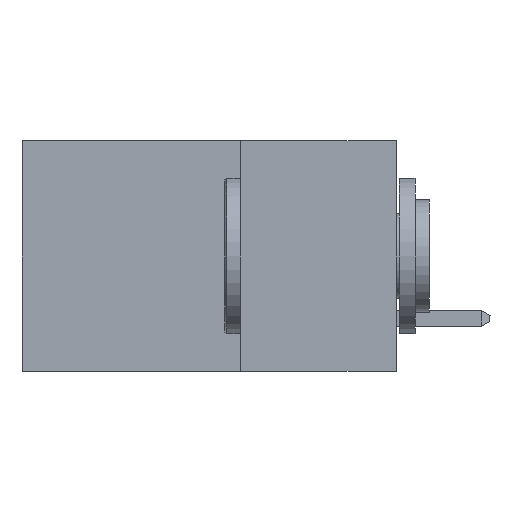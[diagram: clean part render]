
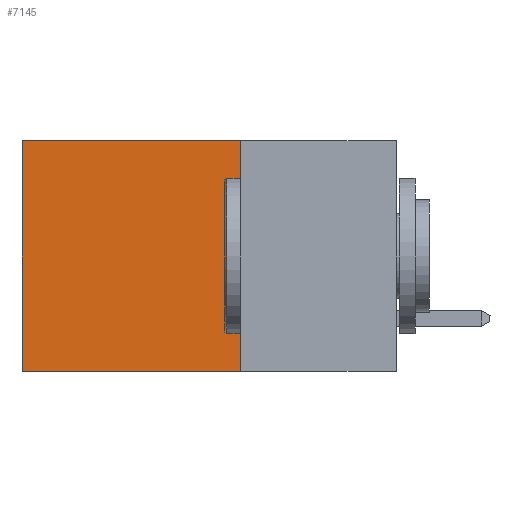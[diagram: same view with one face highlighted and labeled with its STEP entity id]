
A CAD part, left-side view. The second image highlights one B-rep face of the part: STEP entity #7145.
In plain terms, the highlighted planar face has unit normal (-1, 0, 0).
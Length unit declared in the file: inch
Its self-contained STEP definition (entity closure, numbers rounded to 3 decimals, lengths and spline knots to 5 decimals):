
#646 = DIRECTION ( 'NONE',  ( 0., 0., -1. ) ) ;
#692 = LINE ( 'NONE', #9301, #15284 ) ;
#779 = EDGE_LOOP ( 'NONE', ( #11069, #17804, #13193, #9553 ) ) ;
#2075 = DIRECTION ( 'NONE',  ( 1., 0., 0. ) ) ;
#2121 = CARTESIAN_POINT ( 'NONE',  ( 0.2615, 0.25, -0.37 ) ) ;
#2460 = CARTESIAN_POINT ( 'NONE',  ( 0.2615, 0.25, 0. ) ) ;
#3595 = VERTEX_POINT ( 'NONE', #14564 ) ;
#4343 = EDGE_CURVE ( 'NONE', #7338, #3595, #5916, .T. ) ;
#4880 = FACE_OUTER_BOUND ( 'NONE', #779, .T. ) ;
#5154 = CARTESIAN_POINT ( 'NONE',  ( 0.2615, 0.25, 0. ) ) ;
#5197 = DIRECTION ( 'NONE',  ( 0., 1., 0. ) ) ;
#5916 = LINE ( 'NONE', #5154, #16550 ) ;
#7145 = ADVANCED_FACE ( 'NONE', ( #4880 ), #9193, .F. ) ;
#7338 = VERTEX_POINT ( 'NONE', #2460 ) ;
#8020 = VERTEX_POINT ( 'NONE', #17848 ) ;
#8502 = AXIS2_PLACEMENT_3D ( 'NONE', #10619, #2075, #11993 ) ;
#9193 = PLANE ( 'NONE',  #8502 ) ;
#9301 = CARTESIAN_POINT ( 'NONE',  ( 0.2615, 0.6, -0.37 ) ) ;
#9553 = ORIENTED_EDGE ( 'NONE', *, *, #4343, .T. ) ;
#9695 = EDGE_CURVE ( 'NONE', #7338, #16377, #14678, .T. ) ;
#10619 = CARTESIAN_POINT ( 'NONE',  ( 0.2615, 0.25, -0.37 ) ) ;
#11069 = ORIENTED_EDGE ( 'NONE', *, *, #14708, .T. ) ;
#11262 = CARTESIAN_POINT ( 'NONE',  ( 0.2615, 0.25, -0.37 ) ) ;
#11478 = VECTOR ( 'NONE', #17130, 39.37008 ) ;
#11899 = LINE ( 'NONE', #15816, #11478 ) ;
#11993 = DIRECTION ( 'NONE',  ( 0., 0., -1. ) ) ;
#12037 = DIRECTION ( 'NONE',  ( 0., 0., -1. ) ) ;
#13193 = ORIENTED_EDGE ( 'NONE', *, *, #9695, .F. ) ;
#13314 = EDGE_CURVE ( 'NONE', #16377, #8020, #11899, .T. ) ;
#14564 = CARTESIAN_POINT ( 'NONE',  ( 0.2615, 0.6, 0. ) ) ;
#14678 = LINE ( 'NONE', #2121, #17377 ) ;
#14708 = EDGE_CURVE ( 'NONE', #3595, #8020, #692, .T. ) ;
#15284 = VECTOR ( 'NONE', #646, 39.37008 ) ;
#15816 = CARTESIAN_POINT ( 'NONE',  ( 0.2615, 0.25, -0.37 ) ) ;
#16377 = VERTEX_POINT ( 'NONE', #11262 ) ;
#16550 = VECTOR ( 'NONE', #5197, 39.37008 ) ;
#17130 = DIRECTION ( 'NONE',  ( 0., 1., 0. ) ) ;
#17377 = VECTOR ( 'NONE', #12037, 39.37008 ) ;
#17804 = ORIENTED_EDGE ( 'NONE', *, *, #13314, .F. ) ;
#17848 = CARTESIAN_POINT ( 'NONE',  ( 0.2615, 0.6, -0.37 ) ) ;
